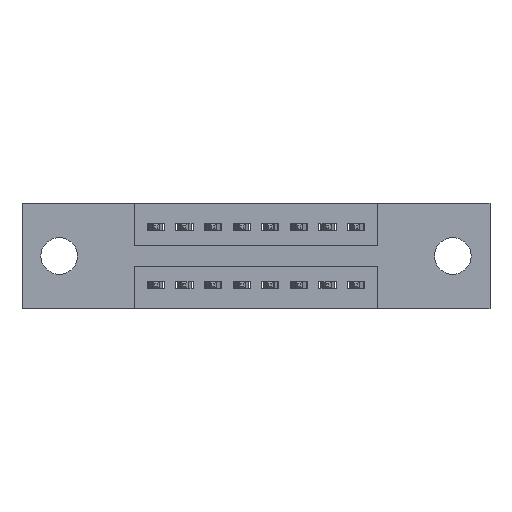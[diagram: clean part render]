
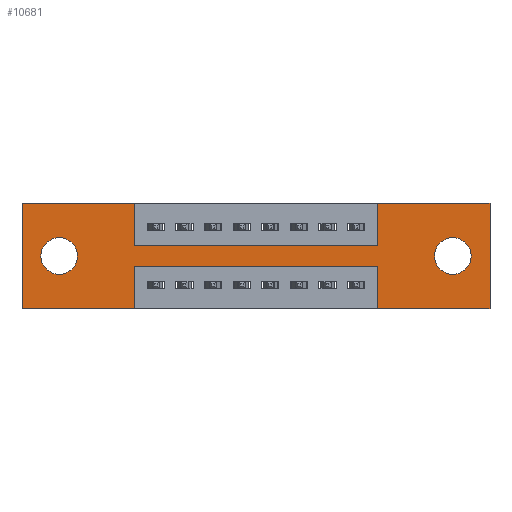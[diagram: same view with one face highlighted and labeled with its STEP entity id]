
A CAD part, front view. The second image highlights one B-rep face of the part: STEP entity #10681.
In plain terms, the highlighted planar face has unit normal (0, -1, 0).
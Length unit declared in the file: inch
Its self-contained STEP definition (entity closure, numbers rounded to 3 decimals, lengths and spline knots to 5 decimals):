
#141 = CARTESIAN_POINT ( 'NONE',  ( 0.13, 0., -0.121 ) ) ;
#221 = FACE_OUTER_BOUND ( 'NONE', #497, .T. ) ;
#332 = DIRECTION ( 'NONE',  ( 0., 0., 1. ) ) ;
#398 = CARTESIAN_POINT ( 'NONE',  ( 1.635, 0., 0. ) ) ;
#497 = EDGE_LOOP ( 'NONE', ( #3185, #1225, #3458, #4021, #4300, #10279, #5946, #7018, #8634, #2238, #9650, #5434 ) ) ;
#542 = LINE ( 'NONE', #5981, #4836 ) ;
#633 = DIRECTION ( 'NONE',  ( 0., 0., 1. ) ) ;
#922 = VERTEX_POINT ( 'NONE', #398 ) ;
#926 = CARTESIAN_POINT ( 'NONE',  ( 0.3925, 0., -0.15 ) ) ;
#1032 = CIRCLE ( 'NONE', #7934, 0.064 ) ;
#1076 = DIRECTION ( 'NONE',  ( 1., 0., 0. ) ) ;
#1099 = EDGE_CURVE ( 'NONE', #2651, #5769, #9900, .T. ) ;
#1120 = VERTEX_POINT ( 'NONE', #3956 ) ;
#1207 = CARTESIAN_POINT ( 'NONE',  ( 1.505, 0., -0.185 ) ) ;
#1225 = ORIENTED_EDGE ( 'NONE', *, *, #9674, .F. ) ;
#1242 = CARTESIAN_POINT ( 'NONE',  ( 0.3925, 0., -0.22 ) ) ;
#1265 = CARTESIAN_POINT ( 'NONE',  ( 0., 0., -0.37 ) ) ;
#1305 = CARTESIAN_POINT ( 'NONE',  ( 0.13, 0., -0.185 ) ) ;
#1338 = VECTOR ( 'NONE', #10087, 39.37008 ) ;
#1351 = EDGE_CURVE ( 'NONE', #922, #5695, #4751, .T. ) ;
#1357 = VECTOR ( 'NONE', #7346, 39.37008 ) ;
#1543 = LINE ( 'NONE', #2844, #1787 ) ;
#1590 = LINE ( 'NONE', #2611, #1338 ) ;
#1598 = VECTOR ( 'NONE', #8070, 39.37008 ) ;
#1604 = ORIENTED_EDGE ( 'NONE', *, *, #9669, .T. ) ;
#1666 = LINE ( 'NONE', #926, #10394 ) ;
#1787 = VECTOR ( 'NONE', #8923, 39.37008 ) ;
#1802 = LINE ( 'NONE', #4565, #10513 ) ;
#1819 = CIRCLE ( 'NONE', #4688, 0.064 ) ;
#1828 = CARTESIAN_POINT ( 'NONE',  ( 0.3925, 0., -0.37 ) ) ;
#1998 = DIRECTION ( 'NONE',  ( 0., 0., -1. ) ) ;
#2004 = CARTESIAN_POINT ( 'NONE',  ( 0.13, 0., -0.185 ) ) ;
#2042 = DIRECTION ( 'NONE',  ( 0., 1., 0. ) ) ;
#2054 = VERTEX_POINT ( 'NONE', #6359 ) ;
#2099 = DIRECTION ( 'NONE',  ( 0., 0., 1. ) ) ;
#2226 = VECTOR ( 'NONE', #8053, 39.37008 ) ;
#2238 = ORIENTED_EDGE ( 'NONE', *, *, #3327, .F. ) ;
#2278 = CARTESIAN_POINT ( 'NONE',  ( 1.635, 0., 0. ) ) ;
#2400 = VECTOR ( 'NONE', #6914, 39.37008 ) ;
#2436 = FACE_BOUND ( 'NONE', #9469, .T. ) ;
#2611 = CARTESIAN_POINT ( 'NONE',  ( 0., 0., 0. ) ) ;
#2651 = VERTEX_POINT ( 'NONE', #9844 ) ;
#2844 = CARTESIAN_POINT ( 'NONE',  ( 1.2425, 0., 0. ) ) ;
#2880 = DIRECTION ( 'NONE',  ( -1., 0., 0. ) ) ;
#2998 = VERTEX_POINT ( 'NONE', #9452 ) ;
#3185 = ORIENTED_EDGE ( 'NONE', *, *, #6733, .F. ) ;
#3327 = EDGE_CURVE ( 'NONE', #5618, #5498, #542, .T. ) ;
#3366 = EDGE_CURVE ( 'NONE', #4634, #4134, #4575, .T. ) ;
#3458 = ORIENTED_EDGE ( 'NONE', *, *, #3366, .F. ) ;
#3625 = LINE ( 'NONE', #10626, #1357 ) ;
#3657 = CARTESIAN_POINT ( 'NONE',  ( 0.3925, 0., 0. ) ) ;
#3713 = EDGE_CURVE ( 'NONE', #4649, #922, #1590, .T. ) ;
#3956 = CARTESIAN_POINT ( 'NONE',  ( 0.3925, 0., -0.22 ) ) ;
#4021 = ORIENTED_EDGE ( 'NONE', *, *, #10521, .F. ) ;
#4117 = ORIENTED_EDGE ( 'NONE', *, *, #8397, .T. ) ;
#4134 = VERTEX_POINT ( 'NONE', #10476 ) ;
#4300 = ORIENTED_EDGE ( 'NONE', *, *, #1351, .F. ) ;
#4530 = VERTEX_POINT ( 'NONE', #7716 ) ;
#4537 = CARTESIAN_POINT ( 'NONE',  ( 1.2425, 0., 0. ) ) ;
#4565 = CARTESIAN_POINT ( 'NONE',  ( 0., 0., -0.37 ) ) ;
#4575 = LINE ( 'NONE', #9545, #2226 ) ;
#4616 = CARTESIAN_POINT ( 'NONE',  ( 0., 0., 0. ) ) ;
#4634 = VERTEX_POINT ( 'NONE', #8706 ) ;
#4649 = VERTEX_POINT ( 'NONE', #4537 ) ;
#4688 = AXIS2_PLACEMENT_3D ( 'NONE', #1207, #7259, #1998 ) ;
#4751 = LINE ( 'NONE', #2278, #2400 ) ;
#4836 = VECTOR ( 'NONE', #1076, 39.37008 ) ;
#4976 = VERTEX_POINT ( 'NONE', #1828 ) ;
#5434 = ORIENTED_EDGE ( 'NONE', *, *, #6068, .F. ) ;
#5465 = DIRECTION ( 'NONE',  ( -1., 0., 0. ) ) ;
#5476 = CARTESIAN_POINT ( 'NONE',  ( 0., 0., 0. ) ) ;
#5498 = VERTEX_POINT ( 'NONE', #3657 ) ;
#5618 = VERTEX_POINT ( 'NONE', #5476 ) ;
#5678 = DIRECTION ( 'NONE',  ( 0., 0., -1. ) ) ;
#5695 = VERTEX_POINT ( 'NONE', #8699 ) ;
#5769 = VERTEX_POINT ( 'NONE', #141 ) ;
#5912 = VERTEX_POINT ( 'NONE', #1265 ) ;
#5946 = ORIENTED_EDGE ( 'NONE', *, *, #9615, .F. ) ;
#5981 = CARTESIAN_POINT ( 'NONE',  ( 0., 0., 0. ) ) ;
#6068 = EDGE_CURVE ( 'NONE', #4976, #5912, #3625, .T. ) ;
#6221 = LINE ( 'NONE', #7469, #1598 ) ;
#6359 = CARTESIAN_POINT ( 'NONE',  ( 0.3925, 0., -0.15 ) ) ;
#6733 = EDGE_CURVE ( 'NONE', #1120, #4976, #10678, .T. ) ;
#6914 = DIRECTION ( 'NONE',  ( 0., 0., -1. ) ) ;
#6968 = EDGE_CURVE ( 'NONE', #5498, #2054, #6221, .T. ) ;
#7018 = ORIENTED_EDGE ( 'NONE', *, *, #9424, .F. ) ;
#7259 = DIRECTION ( 'NONE',  ( 0., 1., 0. ) ) ;
#7308 = CARTESIAN_POINT ( 'NONE',  ( 1.505, 0., -0.185 ) ) ;
#7346 = DIRECTION ( 'NONE',  ( -1., 0., 0. ) ) ;
#7365 = DIRECTION ( 'NONE',  ( 0., 1., 0. ) ) ;
#7469 = CARTESIAN_POINT ( 'NONE',  ( 0.3925, 0., 0. ) ) ;
#7536 = VERTEX_POINT ( 'NONE', #10835 ) ;
#7553 = EDGE_LOOP ( 'NONE', ( #1604, #10788 ) ) ;
#7669 = VECTOR ( 'NONE', #2880, 39.37008 ) ;
#7716 = CARTESIAN_POINT ( 'NONE',  ( 1.505, 0., -0.249 ) ) ;
#7934 = AXIS2_PLACEMENT_3D ( 'NONE', #7308, #2042, #8176 ) ;
#7944 = LINE ( 'NONE', #1242, #7669 ) ;
#7974 = CIRCLE ( 'NONE', #9271, 0.064 ) ;
#7983 = DIRECTION ( 'NONE',  ( 0., 0., -1. ) ) ;
#8053 = DIRECTION ( 'NONE',  ( 0., 0., 1. ) ) ;
#8070 = DIRECTION ( 'NONE',  ( 0., 0., -1. ) ) ;
#8176 = DIRECTION ( 'NONE',  ( 0., 0., -1. ) ) ;
#8215 = AXIS2_PLACEMENT_3D ( 'NONE', #9840, #10584, #5678 ) ;
#8254 = PLANE ( 'NONE',  #8215 ) ;
#8299 = EDGE_CURVE ( 'NONE', #4530, #7536, #1819, .T. ) ;
#8321 = EDGE_CURVE ( 'NONE', #5912, #5618, #10762, .T. ) ;
#8387 = VECTOR ( 'NONE', #7983, 39.37008 ) ;
#8397 = EDGE_CURVE ( 'NONE', #5769, #2651, #7974, .T. ) ;
#8484 = VECTOR ( 'NONE', #332, 39.37008 ) ;
#8495 = AXIS2_PLACEMENT_3D ( 'NONE', #2004, #10393, #633 ) ;
#8634 = ORIENTED_EDGE ( 'NONE', *, *, #6968, .F. ) ;
#8676 = CARTESIAN_POINT ( 'NONE',  ( 0.3925, 0., -0.37 ) ) ;
#8699 = CARTESIAN_POINT ( 'NONE',  ( 1.635, 0., -0.37 ) ) ;
#8706 = CARTESIAN_POINT ( 'NONE',  ( 1.2425, 0., -0.37 ) ) ;
#8923 = DIRECTION ( 'NONE',  ( 0., 0., 1. ) ) ;
#9271 = AXIS2_PLACEMENT_3D ( 'NONE', #1305, #7365, #2099 ) ;
#9424 = EDGE_CURVE ( 'NONE', #2054, #2998, #1666, .T. ) ;
#9438 = DIRECTION ( 'NONE',  ( 1., 0., 0. ) ) ;
#9452 = CARTESIAN_POINT ( 'NONE',  ( 1.2425, 0., -0.15 ) ) ;
#9469 = EDGE_LOOP ( 'NONE', ( #4117, #10079 ) ) ;
#9545 = CARTESIAN_POINT ( 'NONE',  ( 1.2425, 0., -0.37 ) ) ;
#9583 = FACE_BOUND ( 'NONE', #7553, .T. ) ;
#9615 = EDGE_CURVE ( 'NONE', #2998, #4649, #1543, .T. ) ;
#9650 = ORIENTED_EDGE ( 'NONE', *, *, #8321, .F. ) ;
#9669 = EDGE_CURVE ( 'NONE', #7536, #4530, #1032, .T. ) ;
#9674 = EDGE_CURVE ( 'NONE', #4134, #1120, #7944, .T. ) ;
#9840 = CARTESIAN_POINT ( 'NONE',  ( 0., 0., -0.37 ) ) ;
#9844 = CARTESIAN_POINT ( 'NONE',  ( 0.13, 0., -0.249 ) ) ;
#9900 = CIRCLE ( 'NONE', #8495, 0.064 ) ;
#10079 = ORIENTED_EDGE ( 'NONE', *, *, #1099, .T. ) ;
#10087 = DIRECTION ( 'NONE',  ( 1., 0., 0. ) ) ;
#10279 = ORIENTED_EDGE ( 'NONE', *, *, #3713, .F. ) ;
#10393 = DIRECTION ( 'NONE',  ( 0., 1., 0. ) ) ;
#10394 = VECTOR ( 'NONE', #9438, 39.37008 ) ;
#10476 = CARTESIAN_POINT ( 'NONE',  ( 1.2425, 0., -0.22 ) ) ;
#10513 = VECTOR ( 'NONE', #5465, 39.37008 ) ;
#10521 = EDGE_CURVE ( 'NONE', #5695, #4634, #1802, .T. ) ;
#10584 = DIRECTION ( 'NONE',  ( 0., -1., 0. ) ) ;
#10626 = CARTESIAN_POINT ( 'NONE',  ( 0., 0., -0.37 ) ) ;
#10678 = LINE ( 'NONE', #8676, #8387 ) ;
#10681 = ADVANCED_FACE ( 'NONE', ( #9583, #2436, #221 ), #8254, .T. ) ;
#10762 = LINE ( 'NONE', #4616, #8484 ) ;
#10788 = ORIENTED_EDGE ( 'NONE', *, *, #8299, .T. ) ;
#10835 = CARTESIAN_POINT ( 'NONE',  ( 1.505, 0., -0.121 ) ) ;
